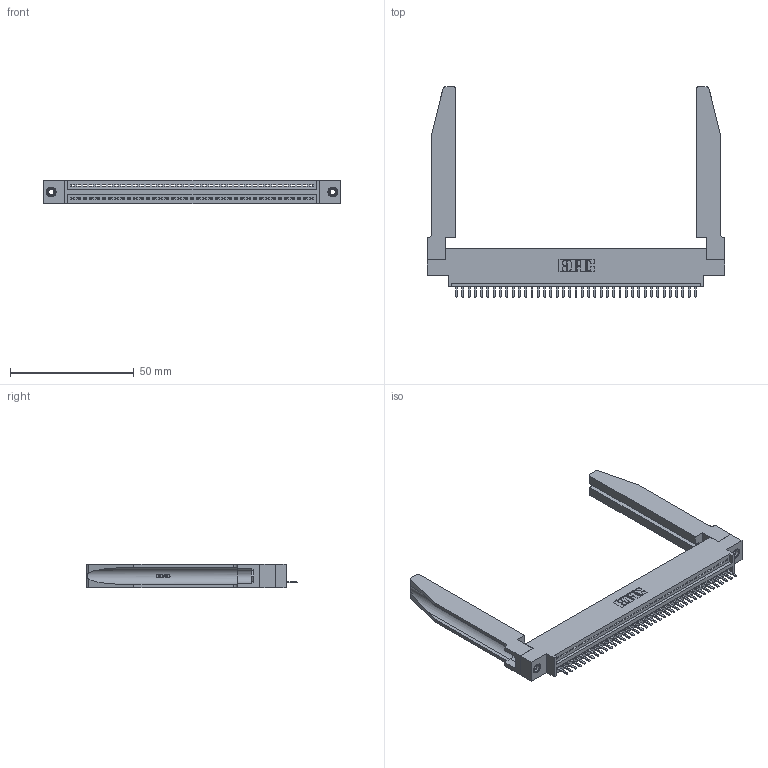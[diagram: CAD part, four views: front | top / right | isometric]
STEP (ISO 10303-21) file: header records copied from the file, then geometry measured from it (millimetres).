
FILE_DESCRIPTION (( 'STEP AP203' ), '1' );
FILE_NAME ('395-039-520-678.STEP', '2019-10-22T02:22:00', ( '' ), ( '' ), 'SwSTEP 2.0', 'SolidWorks 2016', '' );
FILE_SCHEMA (( 'CONFIG_CONTROL_DESIGN' ));
Length unit declared in the file: inch
Products named in the file (5): 395-039-520-678; 345 Part_0.170 Offset - 0.156 Dia-TH; 345-220-078_345-220-078; 345-292-001_345-293-120; 345-250-001_345-250-001-102
Assembly tree (44 placements, depth 2):
  395-039-520-678
    345 Part_0.170 Offset - 0.156 Dia-TH
    345-292-001_345-293-120  x39
    345-250-001_345-250-001-102  x2
    345-220-078_345-220-078  x2
Bounding box: 120.29 x 84.96 x 9.4 mm (x, y, z)
Volume: 18946 mm3; surface area: 21415.6 mm2
Topology: 44 solids, 44 shells, 2782 faces, 8137 edges, 5310 vertices
Faces by surface type: plane 1864, cylinder 866, bspline 36, cone 12, torus 4
Entity records: 34742 total; most frequent: CARTESIAN_POINT 6928, ORIENTED_EDGE 5786, DIRECTION 5049, EDGE_CURVE 2893, LINE 2507, VECTOR 2507, VERTEX_POINT 1920, AXIS2_PLACEMENT_3D 1271
